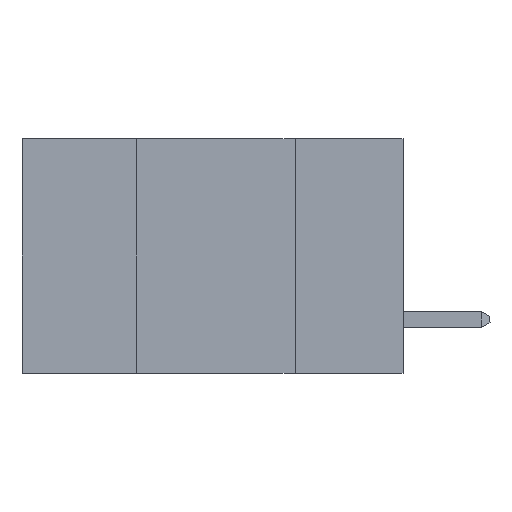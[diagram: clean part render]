
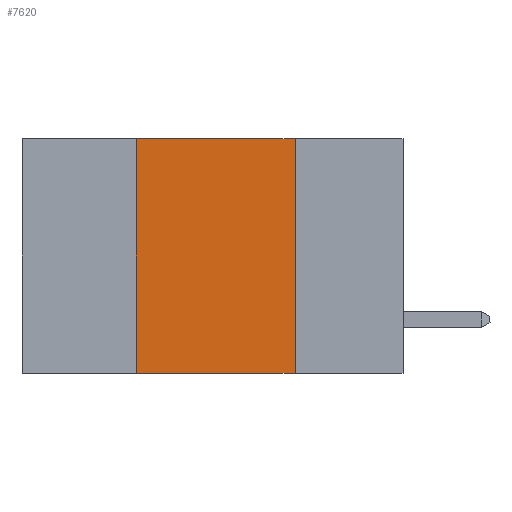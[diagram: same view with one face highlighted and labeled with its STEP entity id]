
A CAD part, left-side view. The second image highlights one B-rep face of the part: STEP entity #7620.
In plain terms, the highlighted planar face has unit normal (-1, 0, 0).
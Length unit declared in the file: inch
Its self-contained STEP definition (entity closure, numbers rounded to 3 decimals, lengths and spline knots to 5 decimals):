
#177 = CARTESIAN_POINT ( 'NONE',  ( 0., 0.42, 0. ) ) ;
#441 = VERTEX_POINT ( 'NONE', #2007 ) ;
#817 = DIRECTION ( 'NONE',  ( 0., 0., -1. ) ) ;
#1324 = CARTESIAN_POINT ( 'NONE',  ( 0., 0.42, -0.37 ) ) ;
#1673 = ORIENTED_EDGE ( 'NONE', *, *, #12695, .F. ) ;
#1728 = CARTESIAN_POINT ( 'NONE',  ( 0., 0.17, 0. ) ) ;
#2007 = CARTESIAN_POINT ( 'NONE',  ( 0., 0.17, 0. ) ) ;
#2074 = LINE ( 'NONE', #177, #11230 ) ;
#2414 = AXIS2_PLACEMENT_3D ( 'NONE', #14058, #7633, #817 ) ;
#2709 = LINE ( 'NONE', #6662, #11148 ) ;
#3115 = PLANE ( 'NONE',  #2414 ) ;
#5154 = CARTESIAN_POINT ( 'NONE',  ( 0., 0.42, 0. ) ) ;
#5345 = CARTESIAN_POINT ( 'NONE',  ( 0., 0.6, -0.37 ) ) ;
#5607 = EDGE_CURVE ( 'NONE', #441, #8325, #13616, .T. ) ;
#6470 = VECTOR ( 'NONE', #12923, 39.37008 ) ;
#6625 = FACE_OUTER_BOUND ( 'NONE', #8152, .T. ) ;
#6662 = CARTESIAN_POINT ( 'NONE',  ( 0., 0.6, 0. ) ) ;
#6896 = CARTESIAN_POINT ( 'NONE',  ( 0., 0.17, -0.37 ) ) ;
#7578 = VECTOR ( 'NONE', #13783, 39.37008 ) ;
#7620 = ADVANCED_FACE ( 'NONE', ( #6625 ), #3115, .F. ) ;
#7633 = DIRECTION ( 'NONE',  ( 1., 0., 0. ) ) ;
#7813 = DIRECTION ( 'NONE',  ( 0., -1., 0. ) ) ;
#8152 = EDGE_LOOP ( 'NONE', ( #8646, #10691, #1673, #10546 ) ) ;
#8177 = DIRECTION ( 'NONE',  ( 0., 0., 1. ) ) ;
#8325 = VERTEX_POINT ( 'NONE', #6896 ) ;
#8646 = ORIENTED_EDGE ( 'NONE', *, *, #5607, .F. ) ;
#9030 = LINE ( 'NONE', #5345, #6470 ) ;
#9898 = EDGE_CURVE ( 'NONE', #11191, #441, #2709, .T. ) ;
#10546 = ORIENTED_EDGE ( 'NONE', *, *, #12952, .T. ) ;
#10691 = ORIENTED_EDGE ( 'NONE', *, *, #9898, .F. ) ;
#11148 = VECTOR ( 'NONE', #7813, 39.37008 ) ;
#11191 = VERTEX_POINT ( 'NONE', #5154 ) ;
#11230 = VECTOR ( 'NONE', #8177, 39.37008 ) ;
#12695 = EDGE_CURVE ( 'NONE', #13641, #11191, #2074, .T. ) ;
#12923 = DIRECTION ( 'NONE',  ( 0., -1., 0. ) ) ;
#12952 = EDGE_CURVE ( 'NONE', #13641, #8325, #9030, .T. ) ;
#13616 = LINE ( 'NONE', #1728, #7578 ) ;
#13641 = VERTEX_POINT ( 'NONE', #1324 ) ;
#13783 = DIRECTION ( 'NONE',  ( 0., 0., -1. ) ) ;
#14058 = CARTESIAN_POINT ( 'NONE',  ( 0., 0.6, 0. ) ) ;
